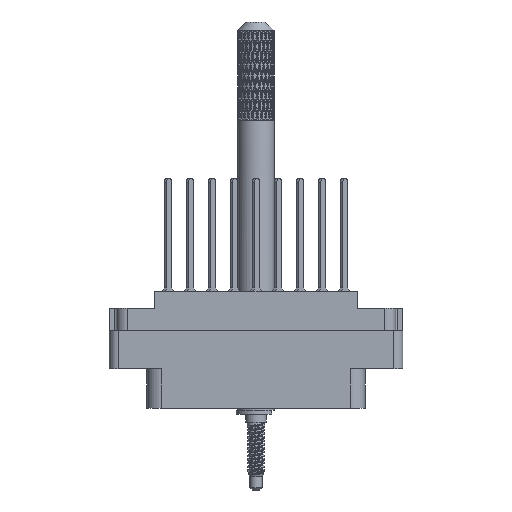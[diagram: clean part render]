
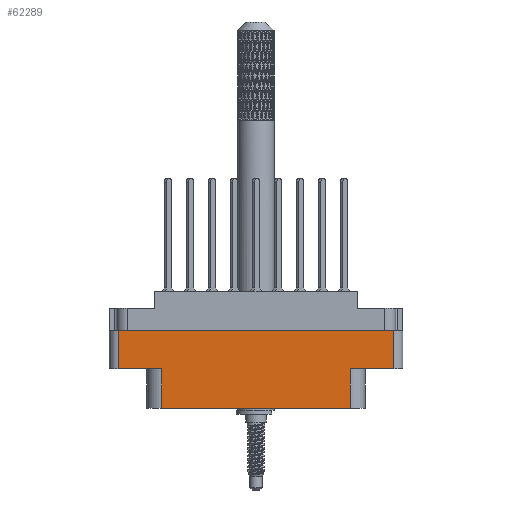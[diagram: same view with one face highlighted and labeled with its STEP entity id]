
A CAD part, front view. The second image highlights one B-rep face of the part: STEP entity #62289.
In plain terms, the highlighted planar face has unit normal (0, -1, 0).
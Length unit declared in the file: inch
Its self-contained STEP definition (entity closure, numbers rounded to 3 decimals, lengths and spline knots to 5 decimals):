
#5220 = ORIENTED_EDGE ( 'NONE', *, *, #82846, .T. ) ;
#8287 = EDGE_LOOP ( 'NONE', ( #73257, #96826, #59021, #10064, #24948, #45686, #88829, #5220 ) ) ;
#10064 = ORIENTED_EDGE ( 'NONE', *, *, #57684, .F. ) ;
#10452 = CARTESIAN_POINT ( 'NONE',  ( -0.938, -0.438, -0.268 ) ) ;
#11529 = EDGE_CURVE ( 'NONE', #76105, #16848, #31896, .T. ) ;
#15431 = DIRECTION ( 'NONE',  ( 0., 0., 1. ) ) ;
#16848 = VERTEX_POINT ( 'NONE', #96303 ) ;
#18634 = LINE ( 'NONE', #79821, #87907 ) ;
#18700 = DIRECTION ( 'NONE',  ( -1., 0., 0. ) ) ;
#19433 = EDGE_CURVE ( 'NONE', #67484, #69975, #18634, .T. ) ;
#21968 = LINE ( 'NONE', #36255, #40516 ) ;
#24948 = ORIENTED_EDGE ( 'NONE', *, *, #60713, .T. ) ;
#25831 = CARTESIAN_POINT ( 'NONE',  ( -1., -0.438, -0.268 ) ) ;
#28686 = LINE ( 'NONE', #33473, #89204 ) ;
#31896 = LINE ( 'NONE', #25831, #81307 ) ;
#32794 = CARTESIAN_POINT ( 'NONE',  ( -0.938, -0.438, -0.798 ) ) ;
#33473 = CARTESIAN_POINT ( 'NONE',  ( -0.938, -0.438, -0.798 ) ) ;
#36255 = CARTESIAN_POINT ( 'NONE',  ( 0.644, -0.438, -0.529 ) ) ;
#37332 = CARTESIAN_POINT ( 'NONE',  ( -0.644, -0.438, -0.529 ) ) ;
#39660 = VECTOR ( 'NONE', #51470, 39.37008 ) ;
#40516 = VECTOR ( 'NONE', #99492, 39.37008 ) ;
#43506 = CARTESIAN_POINT ( 'NONE',  ( 0., -0.438, -0.529 ) ) ;
#45686 = ORIENTED_EDGE ( 'NONE', *, *, #11529, .F. ) ;
#48507 = VERTEX_POINT ( 'NONE', #59476 ) ;
#49072 = LINE ( 'NONE', #72056, #88607 ) ;
#49816 = CARTESIAN_POINT ( 'NONE',  ( 0., -0.438, -0.529 ) ) ;
#51359 = CARTESIAN_POINT ( 'NONE',  ( 0.644, -0.438, -0.529 ) ) ;
#51470 = DIRECTION ( 'NONE',  ( 1., 0., 0. ) ) ;
#55287 = LINE ( 'NONE', #65579, #63860 ) ;
#55702 = LINE ( 'NONE', #43506, #39660 ) ;
#56414 = VERTEX_POINT ( 'NONE', #99765 ) ;
#57538 = DIRECTION ( 'NONE',  ( 1., 0., 0. ) ) ;
#57684 = EDGE_CURVE ( 'NONE', #48507, #77900, #99144, .T. ) ;
#58148 = EDGE_CURVE ( 'NONE', #91487, #76105, #28686, .T. ) ;
#59021 = ORIENTED_EDGE ( 'NONE', *, *, #66009, .F. ) ;
#59476 = CARTESIAN_POINT ( 'NONE',  ( 0.938, -0.438, -0.529 ) ) ;
#60713 = EDGE_CURVE ( 'NONE', #48507, #16848, #49072, .T. ) ;
#62289 = ADVANCED_FACE ( 'NONE', ( #91016 ), #64488, .T. ) ;
#63860 = VECTOR ( 'NONE', #65917, 39.37008 ) ;
#64457 = VECTOR ( 'NONE', #18700, 39.37008 ) ;
#64488 = PLANE ( 'NONE',  #98501 ) ;
#65579 = CARTESIAN_POINT ( 'NONE',  ( -0.938, -0.438, -0.798 ) ) ;
#65860 = DIRECTION ( 'NONE',  ( 0., 0., 1. ) ) ;
#65917 = DIRECTION ( 'NONE',  ( 1., 0., 0. ) ) ;
#66009 = EDGE_CURVE ( 'NONE', #77900, #56414, #21968, .T. ) ;
#67484 = VERTEX_POINT ( 'NONE', #37332 ) ;
#69975 = VERTEX_POINT ( 'NONE', #78480 ) ;
#72056 = CARTESIAN_POINT ( 'NONE',  ( 0.938, -0.438, -0.798 ) ) ;
#73257 = ORIENTED_EDGE ( 'NONE', *, *, #19433, .T. ) ;
#76105 = VERTEX_POINT ( 'NONE', #10452 ) ;
#77900 = VERTEX_POINT ( 'NONE', #51359 ) ;
#78480 = CARTESIAN_POINT ( 'NONE',  ( -0.644, -0.438, -0.798 ) ) ;
#79048 = DIRECTION ( 'NONE',  ( 0., 0., -1. ) ) ;
#79821 = CARTESIAN_POINT ( 'NONE',  ( -0.644, -0.438, -0.529 ) ) ;
#81307 = VECTOR ( 'NONE', #57538, 39.37008 ) ;
#82846 = EDGE_CURVE ( 'NONE', #91487, #67484, #55702, .T. ) ;
#87339 = DIRECTION ( 'NONE',  ( 0., -1., 0. ) ) ;
#87907 = VECTOR ( 'NONE', #88107, 39.37008 ) ;
#88107 = DIRECTION ( 'NONE',  ( 0., 0., -1. ) ) ;
#88607 = VECTOR ( 'NONE', #15431, 39.37008 ) ;
#88829 = ORIENTED_EDGE ( 'NONE', *, *, #58148, .F. ) ;
#89204 = VECTOR ( 'NONE', #65860, 39.37008 ) ;
#91016 = FACE_OUTER_BOUND ( 'NONE', #8287, .T. ) ;
#91487 = VERTEX_POINT ( 'NONE', #92106 ) ;
#92106 = CARTESIAN_POINT ( 'NONE',  ( -0.938, -0.438, -0.529 ) ) ;
#96303 = CARTESIAN_POINT ( 'NONE',  ( 0.938, -0.438, -0.268 ) ) ;
#96826 = ORIENTED_EDGE ( 'NONE', *, *, #97198, .T. ) ;
#97198 = EDGE_CURVE ( 'NONE', #69975, #56414, #55287, .T. ) ;
#98501 = AXIS2_PLACEMENT_3D ( 'NONE', #32794, #87339, #79048 ) ;
#99144 = LINE ( 'NONE', #49816, #64457 ) ;
#99492 = DIRECTION ( 'NONE',  ( 0., 0., -1. ) ) ;
#99765 = CARTESIAN_POINT ( 'NONE',  ( 0.644, -0.438, -0.798 ) ) ;
